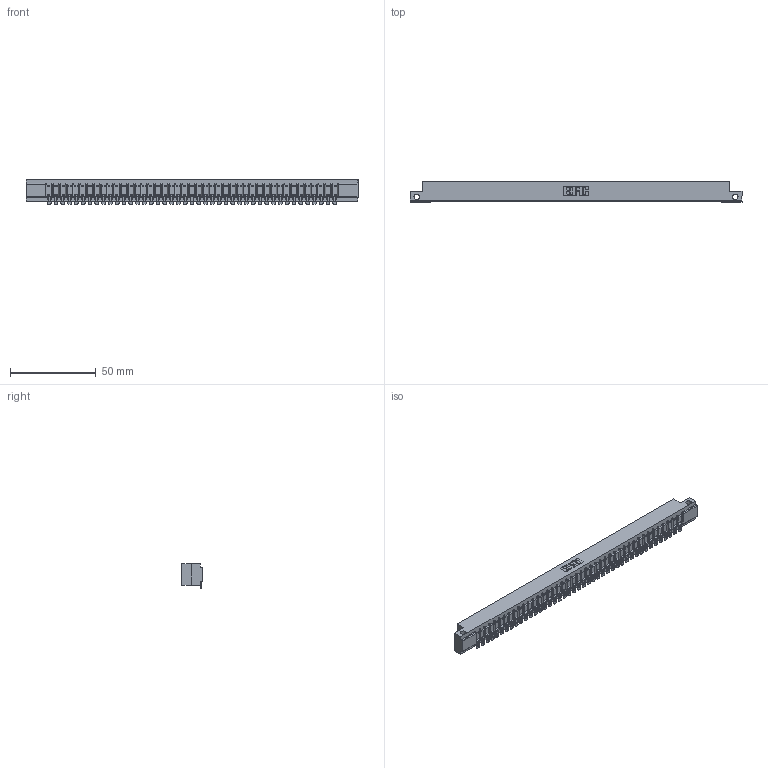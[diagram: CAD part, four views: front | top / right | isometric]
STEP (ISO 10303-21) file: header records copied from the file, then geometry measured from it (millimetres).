
FILE_DESCRIPTION (( 'STEP AP203' ), '1' );
FILE_NAME ('307-043-554-112.STEP', '2018-08-06T01:00:17', ( '' ), ( '' ), 'SwSTEP 2.0', 'SolidWorks 2016', '' );
FILE_SCHEMA (( 'CONFIG_CONTROL_DESIGN' ));
Length unit declared in the file: inch
Products named in the file (3): 307 Part_.128 Dia Side Mounting Holes; 307-290-002_554; 307-043-554-112
Assembly tree (44 placements, depth 2):
  307-043-554-112
    307 Part_.128 Dia Side Mounting Holes
    307-290-002_554  x43
Bounding box: 193.4 x 12.01 x 14.52 mm (x, y, z)
Volume: 20576.6 mm3; surface area: 26048.7 mm2
Topology: 44 solids, 44 shells, 3645 faces, 11202 edges, 7348 vertices
Faces by surface type: plane 2048, cylinder 1509, sphere 88
Entity records: 37707 total; most frequent: CARTESIAN_POINT 6362, ORIENTED_EDGE 6352, DIRECTION 6186, EDGE_CURVE 3176, VECTOR 2426, LINE 2426, VERTEX_POINT 2056, AXIS2_PLACEMENT_3D 1880
